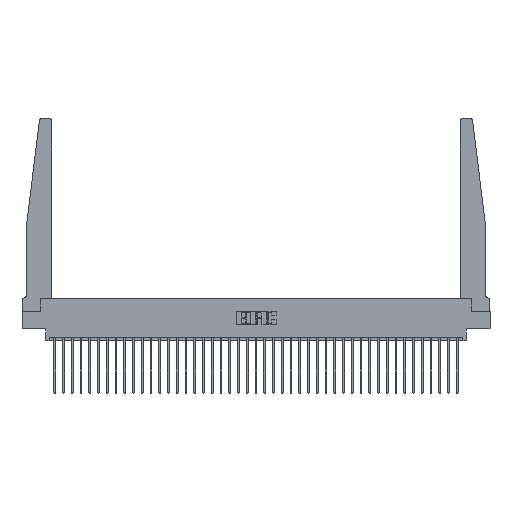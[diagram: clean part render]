
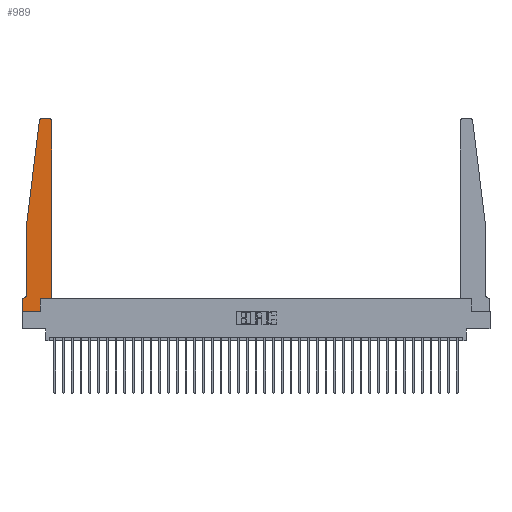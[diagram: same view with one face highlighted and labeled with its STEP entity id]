
A CAD part, top view. The second image highlights one B-rep face of the part: STEP entity #989.
In plain terms, the highlighted planar face has unit normal (0, 0, 1).
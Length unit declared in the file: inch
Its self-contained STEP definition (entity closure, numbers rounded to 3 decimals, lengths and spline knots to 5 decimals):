
#538 = CARTESIAN_POINT ( 'NONE',  ( 0.25, 2.75, 0.37 ) ) ;
#582 = EDGE_CURVE ( 'NONE', #19018, #3067, #24698, .T. ) ;
#740 = DIRECTION ( 'NONE',  ( 0., -1., 0. ) ) ;
#904 = CARTESIAN_POINT ( 'NONE',  ( 0., 0.1875, 0.37 ) ) ;
#989 = ADVANCED_FACE ( 'NONE', ( #20014 ), #9045, .T. ) ;
#1416 = CARTESIAN_POINT ( 'NONE',  ( 0.2605, 0.18, 0.37 ) ) ;
#1430 = VERTEX_POINT ( 'NONE', #32250 ) ;
#1612 = ORIENTED_EDGE ( 'NONE', *, *, #30501, .T. ) ;
#2187 = DIRECTION ( 'NONE',  ( 0., 0., 1. ) ) ;
#2439 = DIRECTION ( 'NONE',  ( 0., -1., 0. ) ) ;
#3067 = VERTEX_POINT ( 'NONE', #1416 ) ;
#3071 = VERTEX_POINT ( 'NONE', #33746 ) ;
#3151 = AXIS2_PLACEMENT_3D ( 'NONE', #6101, #24986, #8802 ) ;
#3215 = DIRECTION ( 'NONE',  ( 0., 1., 0. ) ) ;
#3554 = CIRCLE ( 'NONE', #3151, 0.05 ) ;
#3754 = ORIENTED_EDGE ( 'NONE', *, *, #26155, .T. ) ;
#3851 = LINE ( 'NONE', #22003, #9344 ) ;
#4035 = CARTESIAN_POINT ( 'NONE',  ( 0.425, 0.18, 0.37 ) ) ;
#4036 = DIRECTION ( 'NONE',  ( 0., 0., 1. ) ) ;
#4208 = ORIENTED_EDGE ( 'NONE', *, *, #19443, .T. ) ;
#5470 = ORIENTED_EDGE ( 'NONE', *, *, #29356, .T. ) ;
#5830 = CARTESIAN_POINT ( 'NONE',  ( 0., 0., 0.37 ) ) ;
#5926 = CARTESIAN_POINT ( 'NONE',  ( 0.065, 0.1875, 0.37 ) ) ;
#6101 = CARTESIAN_POINT ( 'NONE',  ( 0.015, 0.2375, 0.37 ) ) ;
#6270 = CARTESIAN_POINT ( 'NONE',  ( 0.015, 0.1875, 0.37 ) ) ;
#6465 = LINE ( 'NONE', #5926, #34274 ) ;
#6574 = VECTOR ( 'NONE', #3215, 39.37008 ) ;
#6743 = EDGE_CURVE ( 'NONE', #26099, #22250, #13756, .T. ) ;
#6981 = CARTESIAN_POINT ( 'NONE',  ( 0.065, 0.2375, 0.37 ) ) ;
#7353 = LINE ( 'NONE', #538, #28852 ) ;
#8640 = DIRECTION ( 'NONE',  ( -1., 0., 0. ) ) ;
#8748 = CIRCLE ( 'NONE', #9664, 0.03 ) ;
#8802 = DIRECTION ( 'NONE',  ( -1., 0., 0. ) ) ;
#9012 = VERTEX_POINT ( 'NONE', #904 ) ;
#9045 = PLANE ( 'NONE',  #33336 ) ;
#9344 = VECTOR ( 'NONE', #13951, 39.37008 ) ;
#9482 = EDGE_CURVE ( 'NONE', #1430, #3071, #7353, .T. ) ;
#9664 = AXIS2_PLACEMENT_3D ( 'NONE', #18419, #2187, #21121 ) ;
#10524 = LINE ( 'NONE', #34758, #18572 ) ;
#10694 = CARTESIAN_POINT ( 'NONE',  ( 0.2605, 0.18, 0.37 ) ) ;
#10838 = CARTESIAN_POINT ( 'NONE',  ( 0.24675, 2.72367, 0.37 ) ) ;
#10945 = ORIENTED_EDGE ( 'NONE', *, *, #22826, .T. ) ;
#11214 = AXIS2_PLACEMENT_3D ( 'NONE', #20226, #4036, #22940 ) ;
#11255 = CARTESIAN_POINT ( 'NONE',  ( 0.425, 0.18, 0.37 ) ) ;
#11338 = DIRECTION ( 'NONE',  ( 0., 1., 0. ) ) ;
#11386 = ORIENTED_EDGE ( 'NONE', *, *, #6743, .T. ) ;
#11743 = LINE ( 'NONE', #4035, #19784 ) ;
#11821 = CIRCLE ( 'NONE', #11214, 0.03 ) ;
#12645 = ORIENTED_EDGE ( 'NONE', *, *, #27947, .T. ) ;
#13756 = LINE ( 'NONE', #11255, #6574 ) ;
#13951 = DIRECTION ( 'NONE',  ( -0.122, -0.992, 0. ) ) ;
#14064 = DIRECTION ( 'NONE',  ( -1., 0., 0. ) ) ;
#14469 = DIRECTION ( 'NONE',  ( 0., 0., 1. ) ) ;
#16495 = EDGE_CURVE ( 'NONE', #22926, #9012, #6465, .T. ) ;
#17077 = CARTESIAN_POINT ( 'NONE',  ( 0.425, 2.72, 0.37 ) ) ;
#18419 = CARTESIAN_POINT ( 'NONE',  ( 0.27653, 2.72, 0.37 ) ) ;
#18572 = VECTOR ( 'NONE', #2439, 39.37008 ) ;
#18767 = EDGE_CURVE ( 'NONE', #9012, #25224, #10524, .T. ) ;
#19018 = VERTEX_POINT ( 'NONE', #34709 ) ;
#19443 = EDGE_CURVE ( 'NONE', #3067, #26099, #11743, .T. ) ;
#19530 = DIRECTION ( 'NONE',  ( 1., 0., 0. ) ) ;
#19784 = VECTOR ( 'NONE', #25513, 39.37008 ) ;
#19876 = VECTOR ( 'NONE', #19530, 39.37008 ) ;
#20014 = FACE_OUTER_BOUND ( 'NONE', #21691, .T. ) ;
#20224 = VERTEX_POINT ( 'NONE', #10838 ) ;
#20226 = CARTESIAN_POINT ( 'NONE',  ( 0.395, 2.72, 0.37 ) ) ;
#21121 = DIRECTION ( 'NONE',  ( 1., 0., 0. ) ) ;
#21691 = EDGE_LOOP ( 'NONE', ( #29941, #3754, #10945, #5470, #12645, #27808, #24518, #1612, #32059, #4208, #11386, #33704 ) ) ;
#22003 = CARTESIAN_POINT ( 'NONE',  ( 0.065, 1.25, 0.37 ) ) ;
#22250 = VERTEX_POINT ( 'NONE', #17077 ) ;
#22733 = VERTEX_POINT ( 'NONE', #29747 ) ;
#22826 = EDGE_CURVE ( 'NONE', #20224, #22733, #3851, .T. ) ;
#22926 = VERTEX_POINT ( 'NONE', #6270 ) ;
#22940 = DIRECTION ( 'NONE',  ( 1., 0., 0. ) ) ;
#24391 = EDGE_CURVE ( 'NONE', #22250, #1430, #11821, .T. ) ;
#24518 = ORIENTED_EDGE ( 'NONE', *, *, #18767, .T. ) ;
#24698 = LINE ( 'NONE', #10694, #25509 ) ;
#24986 = DIRECTION ( 'NONE',  ( 0., 0., -1. ) ) ;
#25224 = VERTEX_POINT ( 'NONE', #5830 ) ;
#25509 = VECTOR ( 'NONE', #11338, 39.37008 ) ;
#25513 = DIRECTION ( 'NONE',  ( 1., 0., 0. ) ) ;
#26099 = VERTEX_POINT ( 'NONE', #26280 ) ;
#26155 = EDGE_CURVE ( 'NONE', #3071, #20224, #8748, .T. ) ;
#26280 = CARTESIAN_POINT ( 'NONE',  ( 0.425, 0.18, 0.37 ) ) ;
#27676 = CARTESIAN_POINT ( 'NONE',  ( 0.065, 1.25, 0.37 ) ) ;
#27808 = ORIENTED_EDGE ( 'NONE', *, *, #16495, .T. ) ;
#27853 = LINE ( 'NONE', #30237, #19876 ) ;
#27889 = CARTESIAN_POINT ( 'NONE',  ( 0., 0.1875, 0.37 ) ) ;
#27947 = EDGE_CURVE ( 'NONE', #28907, #22926, #3554, .T. ) ;
#28852 = VECTOR ( 'NONE', #8640, 39.37008 ) ;
#28907 = VERTEX_POINT ( 'NONE', #6981 ) ;
#29356 = EDGE_CURVE ( 'NONE', #22733, #28907, #32978, .T. ) ;
#29747 = CARTESIAN_POINT ( 'NONE',  ( 0.065, 1.25, 0.37 ) ) ;
#29941 = ORIENTED_EDGE ( 'NONE', *, *, #9482, .T. ) ;
#30237 = CARTESIAN_POINT ( 'NONE',  ( 0., 0., 0.37 ) ) ;
#30501 = EDGE_CURVE ( 'NONE', #25224, #19018, #27853, .T. ) ;
#32059 = ORIENTED_EDGE ( 'NONE', *, *, #582, .T. ) ;
#32165 = VECTOR ( 'NONE', #740, 39.37008 ) ;
#32250 = CARTESIAN_POINT ( 'NONE',  ( 0.395, 2.75, 0.37 ) ) ;
#32978 = LINE ( 'NONE', #27676, #32165 ) ;
#33305 = DIRECTION ( 'NONE',  ( 1., 0., 0. ) ) ;
#33336 = AXIS2_PLACEMENT_3D ( 'NONE', #27889, #14469, #33305 ) ;
#33704 = ORIENTED_EDGE ( 'NONE', *, *, #24391, .T. ) ;
#33746 = CARTESIAN_POINT ( 'NONE',  ( 0.27653, 2.75, 0.37 ) ) ;
#34274 = VECTOR ( 'NONE', #14064, 39.37008 ) ;
#34709 = CARTESIAN_POINT ( 'NONE',  ( 0.2605, 0., 0.37 ) ) ;
#34758 = CARTESIAN_POINT ( 'NONE',  ( 0., 0., 0.37 ) ) ;
